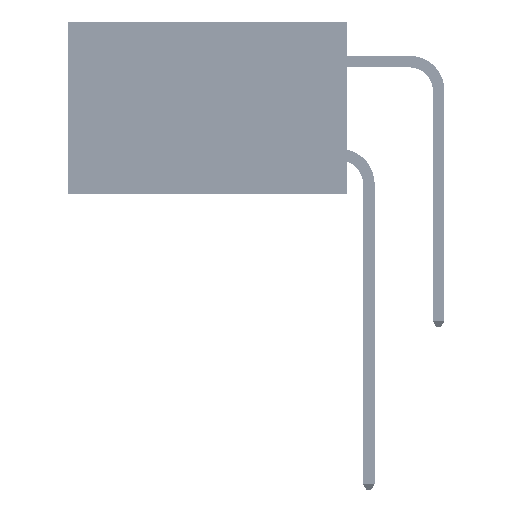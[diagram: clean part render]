
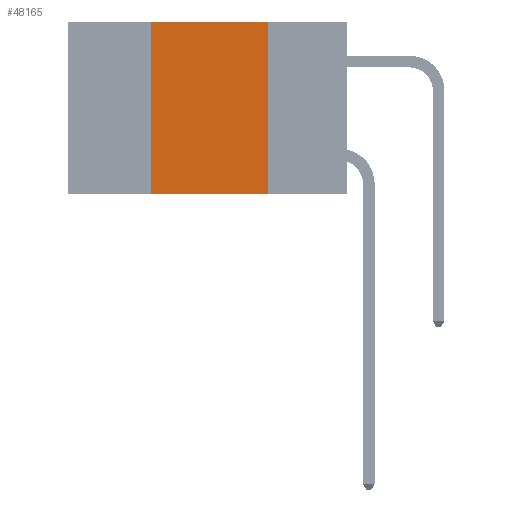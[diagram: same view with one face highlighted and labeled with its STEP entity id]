
A CAD part, left-side view. The second image highlights one B-rep face of the part: STEP entity #48165.
In plain terms, the highlighted planar face has unit normal (-1, 0, 0).
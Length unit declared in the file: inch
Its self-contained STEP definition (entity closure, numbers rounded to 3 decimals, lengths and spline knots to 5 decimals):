
#147 = VERTEX_POINT ( 'NONE', #43236 ) ;
#320 = DIRECTION ( 'NONE',  ( 0., 0., 1. ) ) ;
#828 = VECTOR ( 'NONE', #24221, 39.37008 ) ;
#2374 = VERTEX_POINT ( 'NONE', #32642 ) ;
#3458 = ORIENTED_EDGE ( 'NONE', *, *, #21367, .F. ) ;
#5096 = CARTESIAN_POINT ( 'NONE',  ( 0., 0.17, 0. ) ) ;
#9359 = CARTESIAN_POINT ( 'NONE',  ( 0., 0.6, 0. ) ) ;
#9903 = DIRECTION ( 'NONE',  ( 0., -1., 0. ) ) ;
#13418 = VERTEX_POINT ( 'NONE', #48367 ) ;
#14585 = EDGE_LOOP ( 'NONE', ( #47269, #3458, #34173, #18631 ) ) ;
#14812 = VECTOR ( 'NONE', #320, 39.37008 ) ;
#15473 = DIRECTION ( 'NONE',  ( 0., 0., -1. ) ) ;
#16650 = CARTESIAN_POINT ( 'NONE',  ( 0., 0.17, -0.37 ) ) ;
#18135 = EDGE_CURVE ( 'NONE', #13418, #18172, #38462, .T. ) ;
#18172 = VERTEX_POINT ( 'NONE', #16650 ) ;
#18631 = ORIENTED_EDGE ( 'NONE', *, *, #36225, .T. ) ;
#19527 = CARTESIAN_POINT ( 'NONE',  ( 0., 0.6, 0. ) ) ;
#19717 = VECTOR ( 'NONE', #30423, 39.37008 ) ;
#19801 = AXIS2_PLACEMENT_3D ( 'NONE', #19527, #45197, #15473 ) ;
#21367 = EDGE_CURVE ( 'NONE', #2374, #13418, #31251, .T. ) ;
#21822 = EDGE_CURVE ( 'NONE', #147, #2374, #24753, .T. ) ;
#24221 = DIRECTION ( 'NONE',  ( 0., -1., 0. ) ) ;
#24753 = LINE ( 'NONE', #38065, #14812 ) ;
#26775 = FACE_OUTER_BOUND ( 'NONE', #14585, .T. ) ;
#26784 = PLANE ( 'NONE',  #19801 ) ;
#30423 = DIRECTION ( 'NONE',  ( 0., 0., -1. ) ) ;
#31251 = LINE ( 'NONE', #9359, #828 ) ;
#32312 = CARTESIAN_POINT ( 'NONE',  ( 0., 0.6, -0.37 ) ) ;
#32642 = CARTESIAN_POINT ( 'NONE',  ( 0., 0.42, 0. ) ) ;
#34173 = ORIENTED_EDGE ( 'NONE', *, *, #21822, .F. ) ;
#36225 = EDGE_CURVE ( 'NONE', #147, #18172, #39865, .T. ) ;
#36357 = VECTOR ( 'NONE', #9903, 39.37008 ) ;
#38065 = CARTESIAN_POINT ( 'NONE',  ( 0., 0.42, 0. ) ) ;
#38462 = LINE ( 'NONE', #5096, #19717 ) ;
#39865 = LINE ( 'NONE', #32312, #36357 ) ;
#43236 = CARTESIAN_POINT ( 'NONE',  ( 0., 0.42, -0.37 ) ) ;
#45197 = DIRECTION ( 'NONE',  ( 1., 0., 0. ) ) ;
#47269 = ORIENTED_EDGE ( 'NONE', *, *, #18135, .F. ) ;
#48165 = ADVANCED_FACE ( 'NONE', ( #26775 ), #26784, .F. ) ;
#48367 = CARTESIAN_POINT ( 'NONE',  ( 0., 0.17, 0. ) ) ;
